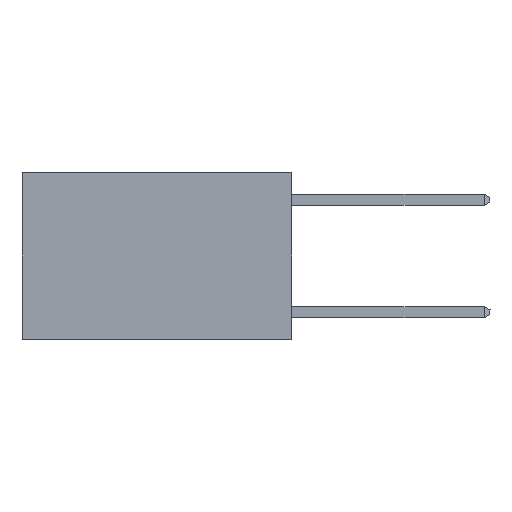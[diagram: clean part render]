
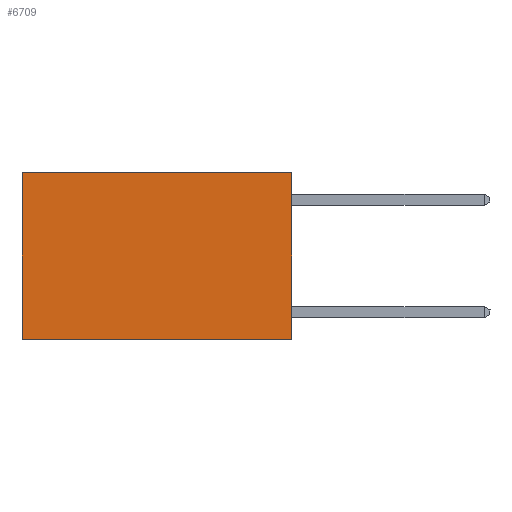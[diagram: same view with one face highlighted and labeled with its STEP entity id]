
A CAD part, left-side view. The second image highlights one B-rep face of the part: STEP entity #6709.
In plain terms, the highlighted planar face has unit normal (-1, 0, 0).
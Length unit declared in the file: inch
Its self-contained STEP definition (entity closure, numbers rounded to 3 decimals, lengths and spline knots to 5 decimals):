
#106 = CARTESIAN_POINT ( 'NONE',  ( 0.2625, 0., 0. ) ) ;
#180 = EDGE_CURVE ( 'NONE', #10385, #8455, #5621, .T. ) ;
#454 = EDGE_CURVE ( 'NONE', #10385, #12699, #15168, .T. ) ;
#1154 = EDGE_LOOP ( 'NONE', ( #1358, #4950, #13741, #14387 ) ) ;
#1358 = ORIENTED_EDGE ( 'NONE', *, *, #11412, .T. ) ;
#1708 = PLANE ( 'NONE',  #9184 ) ;
#1830 = CARTESIAN_POINT ( 'NONE',  ( 0.2625, 0.6, 0. ) ) ;
#1886 = DIRECTION ( 'NONE',  ( 0., 1., 0. ) ) ;
#3018 = LINE ( 'NONE', #1830, #7860 ) ;
#4884 = VECTOR ( 'NONE', #1886, 39.37008 ) ;
#4950 = ORIENTED_EDGE ( 'NONE', *, *, #8317, .F. ) ;
#5596 = CARTESIAN_POINT ( 'NONE',  ( 0.2625, 0., 0. ) ) ;
#5621 = LINE ( 'NONE', #106, #10342 ) ;
#5842 = CARTESIAN_POINT ( 'NONE',  ( 0.2625, 0., -0.37 ) ) ;
#6167 = LINE ( 'NONE', #5842, #12443 ) ;
#6709 = ADVANCED_FACE ( 'NONE', ( #13384 ), #1708, .F. ) ;
#6907 = DIRECTION ( 'NONE',  ( 0., 0., -1. ) ) ;
#7860 = VECTOR ( 'NONE', #6907, 39.37008 ) ;
#8317 = EDGE_CURVE ( 'NONE', #8455, #13175, #6167, .T. ) ;
#8455 = VERTEX_POINT ( 'NONE', #10153 ) ;
#9184 = AXIS2_PLACEMENT_3D ( 'NONE', #5596, #14563, #14735 ) ;
#10153 = CARTESIAN_POINT ( 'NONE',  ( 0.2625, 0., -0.37 ) ) ;
#10342 = VECTOR ( 'NONE', #15859, 39.37008 ) ;
#10385 = VERTEX_POINT ( 'NONE', #10784 ) ;
#10784 = CARTESIAN_POINT ( 'NONE',  ( 0.2625, 0., 0. ) ) ;
#11365 = DIRECTION ( 'NONE',  ( 0., 1., 0. ) ) ;
#11412 = EDGE_CURVE ( 'NONE', #12699, #13175, #3018, .T. ) ;
#11957 = CARTESIAN_POINT ( 'NONE',  ( 0.2625, 0.6, 0. ) ) ;
#12443 = VECTOR ( 'NONE', #11365, 39.37008 ) ;
#12699 = VERTEX_POINT ( 'NONE', #11957 ) ;
#13175 = VERTEX_POINT ( 'NONE', #16363 ) ;
#13384 = FACE_OUTER_BOUND ( 'NONE', #1154, .T. ) ;
#13741 = ORIENTED_EDGE ( 'NONE', *, *, #180, .F. ) ;
#14387 = ORIENTED_EDGE ( 'NONE', *, *, #454, .T. ) ;
#14563 = DIRECTION ( 'NONE',  ( 1., 0., 0. ) ) ;
#14735 = DIRECTION ( 'NONE',  ( 0., 0., -1. ) ) ;
#15168 = LINE ( 'NONE', #16178, #4884 ) ;
#15859 = DIRECTION ( 'NONE',  ( 0., 0., -1. ) ) ;
#16178 = CARTESIAN_POINT ( 'NONE',  ( 0.2625, 0., 0. ) ) ;
#16363 = CARTESIAN_POINT ( 'NONE',  ( 0.2625, 0.6, -0.37 ) ) ;
